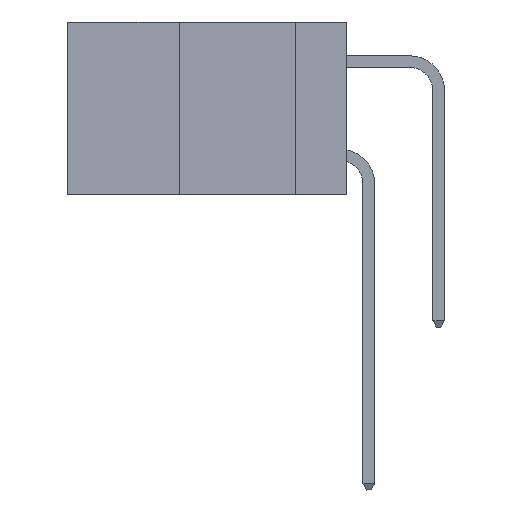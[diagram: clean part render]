
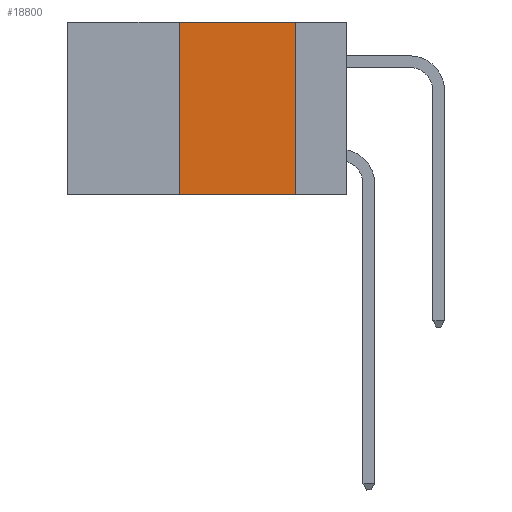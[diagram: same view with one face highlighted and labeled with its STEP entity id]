
A CAD part, left-side view. The second image highlights one B-rep face of the part: STEP entity #18800.
In plain terms, the highlighted planar face has unit normal (-1, 0, 0).
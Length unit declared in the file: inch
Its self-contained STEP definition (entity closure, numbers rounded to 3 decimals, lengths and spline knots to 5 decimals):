
#218 = ORIENTED_EDGE ( 'NONE', *, *, #3986, .F. ) ;
#359 = ORIENTED_EDGE ( 'NONE', *, *, #12769, .F. ) ;
#636 = VERTEX_POINT ( 'NONE', #1371 ) ;
#1371 = CARTESIAN_POINT ( 'NONE',  ( 0., 0.11, 0. ) ) ;
#1496 = LINE ( 'NONE', #14572, #18388 ) ;
#1772 = ORIENTED_EDGE ( 'NONE', *, *, #11831, .F. ) ;
#2247 = VERTEX_POINT ( 'NONE', #14720 ) ;
#3475 = CARTESIAN_POINT ( 'NONE',  ( 0., 0.11, 0. ) ) ;
#3514 = DIRECTION ( 'NONE',  ( 0., 0., -1. ) ) ;
#3928 = VECTOR ( 'NONE', #3514, 39.37008 ) ;
#3986 = EDGE_CURVE ( 'NONE', #636, #17490, #8843, .T. ) ;
#4309 = VERTEX_POINT ( 'NONE', #13286 ) ;
#5024 = DIRECTION ( 'NONE',  ( 0., -1., 0. ) ) ;
#5358 = ORIENTED_EDGE ( 'NONE', *, *, #14228, .T. ) ;
#8107 = VECTOR ( 'NONE', #9883, 39.37008 ) ;
#8589 = LINE ( 'NONE', #16047, #8107 ) ;
#8626 = VECTOR ( 'NONE', #18468, 39.37008 ) ;
#8843 = LINE ( 'NONE', #3475, #3928 ) ;
#9102 = LINE ( 'NONE', #9273, #8626 ) ;
#9273 = CARTESIAN_POINT ( 'NONE',  ( 0., 0.36, 0. ) ) ;
#9680 = CARTESIAN_POINT ( 'NONE',  ( 0., 0.6, 0. ) ) ;
#9883 = DIRECTION ( 'NONE',  ( 0., -1., 0. ) ) ;
#10463 = AXIS2_PLACEMENT_3D ( 'NONE', #9680, #20287, #11222 ) ;
#11222 = DIRECTION ( 'NONE',  ( 0., 0., -1. ) ) ;
#11831 = EDGE_CURVE ( 'NONE', #2247, #4309, #9102, .T. ) ;
#12746 = PLANE ( 'NONE',  #10463 ) ;
#12769 = EDGE_CURVE ( 'NONE', #4309, #636, #8589, .T. ) ;
#13286 = CARTESIAN_POINT ( 'NONE',  ( 0., 0.36, 0. ) ) ;
#14228 = EDGE_CURVE ( 'NONE', #2247, #17490, #1496, .T. ) ;
#14572 = CARTESIAN_POINT ( 'NONE',  ( 0., 0.6, -0.37 ) ) ;
#14720 = CARTESIAN_POINT ( 'NONE',  ( 0., 0.36, -0.37 ) ) ;
#15429 = FACE_OUTER_BOUND ( 'NONE', #15604, .T. ) ;
#15604 = EDGE_LOOP ( 'NONE', ( #218, #359, #1772, #5358 ) ) ;
#16047 = CARTESIAN_POINT ( 'NONE',  ( 0., 0.6, 0. ) ) ;
#17490 = VERTEX_POINT ( 'NONE', #18619 ) ;
#18388 = VECTOR ( 'NONE', #5024, 39.37008 ) ;
#18468 = DIRECTION ( 'NONE',  ( 0., 0., 1. ) ) ;
#18619 = CARTESIAN_POINT ( 'NONE',  ( 0., 0.11, -0.37 ) ) ;
#18800 = ADVANCED_FACE ( 'NONE', ( #15429 ), #12746, .F. ) ;
#20287 = DIRECTION ( 'NONE',  ( 1., 0., 0. ) ) ;
